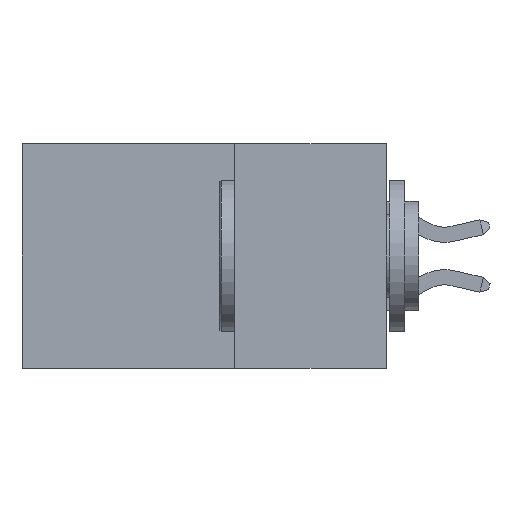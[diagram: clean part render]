
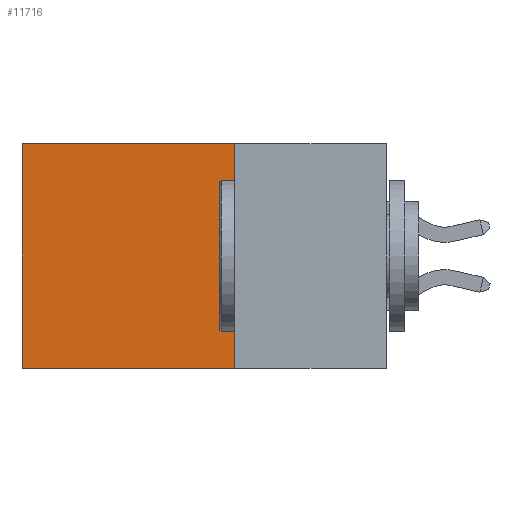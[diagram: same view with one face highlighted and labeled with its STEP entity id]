
A CAD part, left-side view. The second image highlights one B-rep face of the part: STEP entity #11716.
In plain terms, the highlighted planar face has unit normal (-1, 0, 0).
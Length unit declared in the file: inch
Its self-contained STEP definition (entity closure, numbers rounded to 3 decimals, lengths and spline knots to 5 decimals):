
#197 = LINE ( 'NONE', #302, #13558 ) ;
#302 = CARTESIAN_POINT ( 'NONE',  ( 0.298, 0.25, 0. ) ) ;
#516 = EDGE_LOOP ( 'NONE', ( #14952, #11949, #11220, #1087 ) ) ;
#1087 = ORIENTED_EDGE ( 'NONE', *, *, #2185, .T. ) ;
#1261 = DIRECTION ( 'NONE',  ( 1., 0., 0. ) ) ;
#2185 = EDGE_CURVE ( 'NONE', #10751, #10502, #8225, .T. ) ;
#2410 = EDGE_CURVE ( 'NONE', #3365, #11342, #10067, .T. ) ;
#2603 = CARTESIAN_POINT ( 'NONE',  ( 0.298, 0.25, 0. ) ) ;
#3365 = VERTEX_POINT ( 'NONE', #10615 ) ;
#3538 = DIRECTION ( 'NONE',  ( 0., 1., 0. ) ) ;
#3670 = PLANE ( 'NONE',  #10921 ) ;
#4004 = CARTESIAN_POINT ( 'NONE',  ( 0.298, 0.25, -0.37 ) ) ;
#5471 = CARTESIAN_POINT ( 'NONE',  ( 0.298, 0.6, 0. ) ) ;
#7478 = CARTESIAN_POINT ( 'NONE',  ( 0.298, 0.6, 0. ) ) ;
#8100 = VECTOR ( 'NONE', #13703, 39.37008 ) ;
#8225 = LINE ( 'NONE', #11519, #16552 ) ;
#8267 = EDGE_CURVE ( 'NONE', #10751, #3365, #197, .T. ) ;
#9505 = CARTESIAN_POINT ( 'NONE',  ( 0.298, 0.25, 0. ) ) ;
#10067 = LINE ( 'NONE', #4004, #12979 ) ;
#10502 = VERTEX_POINT ( 'NONE', #7478 ) ;
#10602 = DIRECTION ( 'NONE',  ( 0., 0., -1. ) ) ;
#10615 = CARTESIAN_POINT ( 'NONE',  ( 0.298, 0.25, -0.37 ) ) ;
#10751 = VERTEX_POINT ( 'NONE', #9505 ) ;
#10754 = DIRECTION ( 'NONE',  ( 0., 1., 0. ) ) ;
#10921 = AXIS2_PLACEMENT_3D ( 'NONE', #2603, #1261, #10602 ) ;
#11220 = ORIENTED_EDGE ( 'NONE', *, *, #8267, .F. ) ;
#11342 = VERTEX_POINT ( 'NONE', #12823 ) ;
#11519 = CARTESIAN_POINT ( 'NONE',  ( 0.298, 0.25, 0. ) ) ;
#11716 = ADVANCED_FACE ( 'NONE', ( #12955 ), #3670, .F. ) ;
#11949 = ORIENTED_EDGE ( 'NONE', *, *, #2410, .F. ) ;
#12823 = CARTESIAN_POINT ( 'NONE',  ( 0.298, 0.6, -0.37 ) ) ;
#12955 = FACE_OUTER_BOUND ( 'NONE', #516, .T. ) ;
#12979 = VECTOR ( 'NONE', #10754, 39.37008 ) ;
#13558 = VECTOR ( 'NONE', #16642, 39.37008 ) ;
#13703 = DIRECTION ( 'NONE',  ( 0., 0., -1. ) ) ;
#14428 = EDGE_CURVE ( 'NONE', #10502, #11342, #15173, .T. ) ;
#14952 = ORIENTED_EDGE ( 'NONE', *, *, #14428, .T. ) ;
#15173 = LINE ( 'NONE', #5471, #8100 ) ;
#16552 = VECTOR ( 'NONE', #3538, 39.37008 ) ;
#16642 = DIRECTION ( 'NONE',  ( 0., 0., -1. ) ) ;
